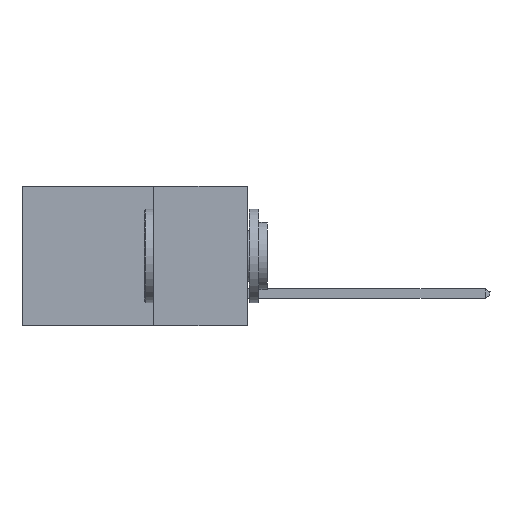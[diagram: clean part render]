
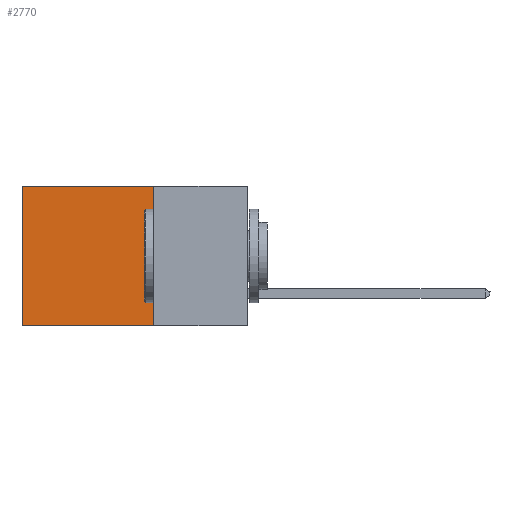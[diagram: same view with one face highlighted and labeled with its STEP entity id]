
A CAD part, left-side view. The second image highlights one B-rep face of the part: STEP entity #2770.
In plain terms, the highlighted planar face has unit normal (-1, 0, 0).
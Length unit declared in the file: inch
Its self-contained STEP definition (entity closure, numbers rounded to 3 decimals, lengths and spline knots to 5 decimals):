
#46 = CARTESIAN_POINT ( 'NONE',  ( 0.2615, 0.6, 0. ) ) ;
#471 = EDGE_LOOP ( 'NONE', ( #7191, #7110, #6773, #6003 ) ) ;
#993 = VECTOR ( 'NONE', #7998, 39.37008 ) ;
#1566 = EDGE_CURVE ( 'NONE', #1587, #3875, #6746, .T. ) ;
#1587 = VERTEX_POINT ( 'NONE', #10631 ) ;
#1748 = CARTESIAN_POINT ( 'NONE',  ( 0.2615, 0.6, -0.37 ) ) ;
#2770 = ADVANCED_FACE ( 'NONE', ( #3888 ), #6599, .F. ) ;
#3063 = EDGE_CURVE ( 'NONE', #11121, #3875, #3565, .T. ) ;
#3565 = LINE ( 'NONE', #1748, #993 ) ;
#3668 = AXIS2_PLACEMENT_3D ( 'NONE', #10124, #11017, #5485 ) ;
#3748 = VECTOR ( 'NONE', #7881, 39.37008 ) ;
#3875 = VERTEX_POINT ( 'NONE', #6224 ) ;
#3888 = FACE_OUTER_BOUND ( 'NONE', #471, .T. ) ;
#4378 = CARTESIAN_POINT ( 'NONE',  ( 0.2615, 0.25, -0.37 ) ) ;
#4556 = EDGE_CURVE ( 'NONE', #8320, #1587, #11255, .T. ) ;
#5303 = CARTESIAN_POINT ( 'NONE',  ( 0.2615, 0.25, 0. ) ) ;
#5485 = DIRECTION ( 'NONE',  ( 0., 0., -1. ) ) ;
#6003 = ORIENTED_EDGE ( 'NONE', *, *, #10663, .T. ) ;
#6108 = LINE ( 'NONE', #5303, #8849 ) ;
#6214 = DIRECTION ( 'NONE',  ( 0., 1., 0. ) ) ;
#6224 = CARTESIAN_POINT ( 'NONE',  ( 0.2615, 0.6, -0.37 ) ) ;
#6599 = PLANE ( 'NONE',  #3668 ) ;
#6746 = LINE ( 'NONE', #7894, #10535 ) ;
#6773 = ORIENTED_EDGE ( 'NONE', *, *, #4556, .F. ) ;
#7110 = ORIENTED_EDGE ( 'NONE', *, *, #1566, .F. ) ;
#7150 = DIRECTION ( 'NONE',  ( 0., 1., 0. ) ) ;
#7191 = ORIENTED_EDGE ( 'NONE', *, *, #3063, .T. ) ;
#7881 = DIRECTION ( 'NONE',  ( 0., 0., -1. ) ) ;
#7894 = CARTESIAN_POINT ( 'NONE',  ( 0.2615, 0.25, -0.37 ) ) ;
#7998 = DIRECTION ( 'NONE',  ( 0., 0., -1. ) ) ;
#8320 = VERTEX_POINT ( 'NONE', #10748 ) ;
#8849 = VECTOR ( 'NONE', #7150, 39.37008 ) ;
#10124 = CARTESIAN_POINT ( 'NONE',  ( 0.2615, 0.25, -0.37 ) ) ;
#10535 = VECTOR ( 'NONE', #6214, 39.37008 ) ;
#10631 = CARTESIAN_POINT ( 'NONE',  ( 0.2615, 0.25, -0.37 ) ) ;
#10663 = EDGE_CURVE ( 'NONE', #8320, #11121, #6108, .T. ) ;
#10748 = CARTESIAN_POINT ( 'NONE',  ( 0.2615, 0.25, 0. ) ) ;
#11017 = DIRECTION ( 'NONE',  ( 1., 0., 0. ) ) ;
#11121 = VERTEX_POINT ( 'NONE', #46 ) ;
#11255 = LINE ( 'NONE', #4378, #3748 ) ;
